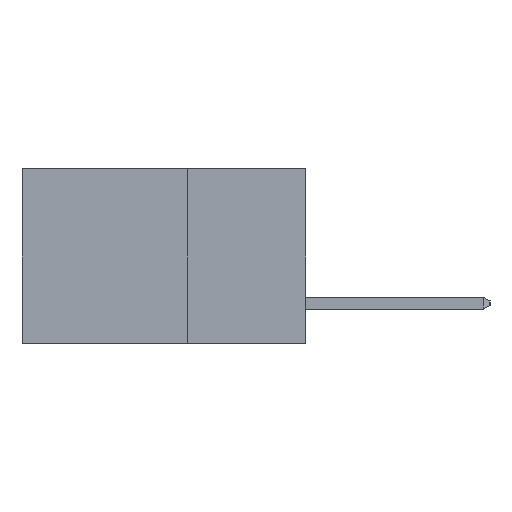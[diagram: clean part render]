
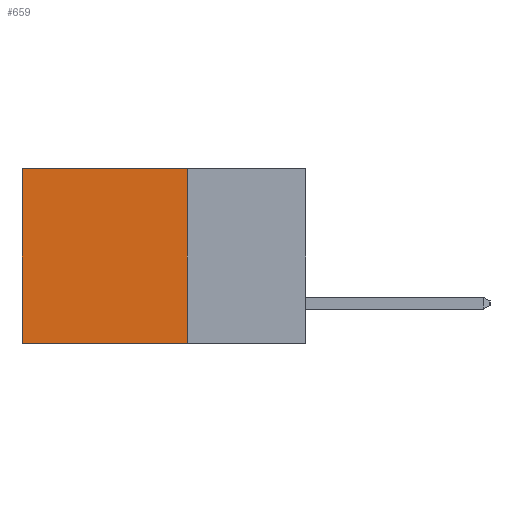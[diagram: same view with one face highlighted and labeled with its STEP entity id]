
A CAD part, left-side view. The second image highlights one B-rep face of the part: STEP entity #659.
In plain terms, the highlighted planar face has unit normal (-1, 0, 0).
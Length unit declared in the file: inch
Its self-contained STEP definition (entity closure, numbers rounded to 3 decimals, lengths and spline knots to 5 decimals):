
#489 = EDGE_CURVE ( 'NONE', #11833, #5429, #3335, .T. ) ;
#659 = ADVANCED_FACE ( 'NONE', ( #3779 ), #4485, .F. ) ;
#1111 = CARTESIAN_POINT ( 'NONE',  ( 0.2615, 0.25, -0.37 ) ) ;
#1208 = LINE ( 'NONE', #1374, #8891 ) ;
#1374 = CARTESIAN_POINT ( 'NONE',  ( 0.2615, 0.6, -0.37 ) ) ;
#1777 = CARTESIAN_POINT ( 'NONE',  ( 0.2615, 0.25, -0.37 ) ) ;
#1838 = DIRECTION ( 'NONE',  ( 0., 0., -1. ) ) ;
#2026 = CARTESIAN_POINT ( 'NONE',  ( 0.2615, 0.25, -0.37 ) ) ;
#2093 = DIRECTION ( 'NONE',  ( 0., 1., 0. ) ) ;
#2277 = CARTESIAN_POINT ( 'NONE',  ( 0.2615, 0.6, 0. ) ) ;
#2362 = DIRECTION ( 'NONE',  ( 0., 1., 0. ) ) ;
#3299 = ORIENTED_EDGE ( 'NONE', *, *, #9469, .T. ) ;
#3335 = LINE ( 'NONE', #10660, #10786 ) ;
#3584 = LINE ( 'NONE', #1777, #5865 ) ;
#3666 = DIRECTION ( 'NONE',  ( 0., 0., -1. ) ) ;
#3779 = FACE_OUTER_BOUND ( 'NONE', #5704, .T. ) ;
#3785 = CARTESIAN_POINT ( 'NONE',  ( 0.2615, 0.6, -0.37 ) ) ;
#4198 = EDGE_CURVE ( 'NONE', #4324, #6311, #5035, .T. ) ;
#4324 = VERTEX_POINT ( 'NONE', #1111 ) ;
#4485 = PLANE ( 'NONE',  #5794 ) ;
#5035 = LINE ( 'NONE', #2026, #12063 ) ;
#5429 = VERTEX_POINT ( 'NONE', #2277 ) ;
#5704 = EDGE_LOOP ( 'NONE', ( #3299, #8736, #12207, #11479 ) ) ;
#5794 = AXIS2_PLACEMENT_3D ( 'NONE', #9751, #10606, #3666 ) ;
#5865 = VECTOR ( 'NONE', #1838, 39.37008 ) ;
#6311 = VERTEX_POINT ( 'NONE', #3785 ) ;
#6495 = EDGE_CURVE ( 'NONE', #11833, #4324, #3584, .T. ) ;
#7901 = CARTESIAN_POINT ( 'NONE',  ( 0.2615, 0.25, 0. ) ) ;
#8120 = DIRECTION ( 'NONE',  ( 0., 0., -1. ) ) ;
#8736 = ORIENTED_EDGE ( 'NONE', *, *, #4198, .F. ) ;
#8891 = VECTOR ( 'NONE', #8120, 39.37008 ) ;
#9469 = EDGE_CURVE ( 'NONE', #5429, #6311, #1208, .T. ) ;
#9751 = CARTESIAN_POINT ( 'NONE',  ( 0.2615, 0.25, -0.37 ) ) ;
#10606 = DIRECTION ( 'NONE',  ( 1., 0., 0. ) ) ;
#10660 = CARTESIAN_POINT ( 'NONE',  ( 0.2615, 0.25, 0. ) ) ;
#10786 = VECTOR ( 'NONE', #2362, 39.37008 ) ;
#11479 = ORIENTED_EDGE ( 'NONE', *, *, #489, .T. ) ;
#11833 = VERTEX_POINT ( 'NONE', #7901 ) ;
#12063 = VECTOR ( 'NONE', #2093, 39.37008 ) ;
#12207 = ORIENTED_EDGE ( 'NONE', *, *, #6495, .F. ) ;
